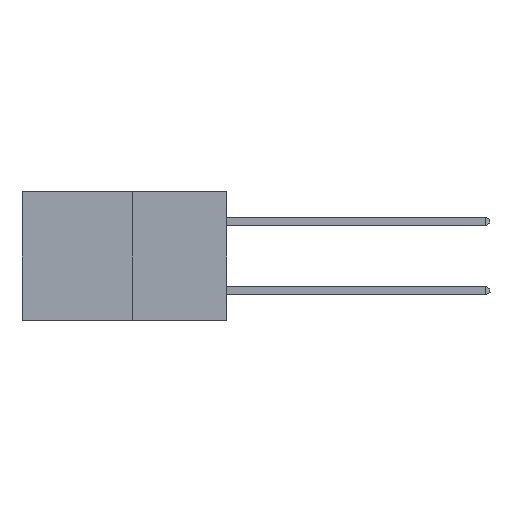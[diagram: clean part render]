
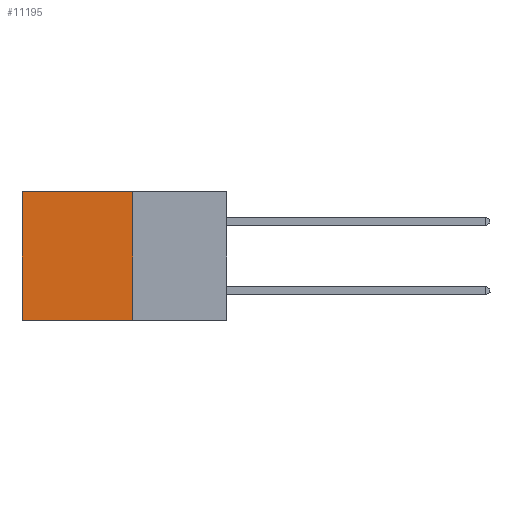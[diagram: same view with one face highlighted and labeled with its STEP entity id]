
A CAD part, left-side view. The second image highlights one B-rep face of the part: STEP entity #11195.
In plain terms, the highlighted planar face has unit normal (-1, 0, 0).
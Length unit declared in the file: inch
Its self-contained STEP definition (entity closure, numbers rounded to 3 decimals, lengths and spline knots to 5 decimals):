
#825 = ORIENTED_EDGE ( 'NONE', *, *, #18292, .T. ) ;
#1033 = LINE ( 'NONE', #4911, #9788 ) ;
#1078 = EDGE_CURVE ( 'NONE', #21351, #6214, #1033, .T. ) ;
#2439 = VERTEX_POINT ( 'NONE', #6594 ) ;
#2441 = LINE ( 'NONE', #10030, #19713 ) ;
#3381 = CARTESIAN_POINT ( 'NONE',  ( 0.277, 0.59, -0.37 ) ) ;
#4911 = CARTESIAN_POINT ( 'NONE',  ( 0.277, 0.27, -0.37 ) ) ;
#5107 = CARTESIAN_POINT ( 'NONE',  ( 0.277, 0.27, 0. ) ) ;
#5161 = DIRECTION ( 'NONE',  ( 0., 1., 0. ) ) ;
#5573 = EDGE_CURVE ( 'NONE', #21214, #2439, #19876, .T. ) ;
#6214 = VERTEX_POINT ( 'NONE', #7865 ) ;
#6594 = CARTESIAN_POINT ( 'NONE',  ( 0.277, 0.59, 0. ) ) ;
#7865 = CARTESIAN_POINT ( 'NONE',  ( 0.277, 0.59, -0.37 ) ) ;
#8168 = PLANE ( 'NONE',  #9071 ) ;
#9071 = AXIS2_PLACEMENT_3D ( 'NONE', #18413, #20121, #9875 ) ;
#9674 = ORIENTED_EDGE ( 'NONE', *, *, #5573, .T. ) ;
#9788 = VECTOR ( 'NONE', #16468, 39.37008 ) ;
#9875 = DIRECTION ( 'NONE',  ( 0., 0., -1. ) ) ;
#10030 = CARTESIAN_POINT ( 'NONE',  ( 0.277, 0.27, -0.37 ) ) ;
#10234 = VECTOR ( 'NONE', #5161, 39.37008 ) ;
#11195 = ADVANCED_FACE ( 'NONE', ( #18753 ), #8168, .F. ) ;
#12161 = DIRECTION ( 'NONE',  ( 0., 0., -1. ) ) ;
#12458 = CARTESIAN_POINT ( 'NONE',  ( 0.277, 0.27, 0. ) ) ;
#12824 = CARTESIAN_POINT ( 'NONE',  ( 0.277, 0.27, -0.37 ) ) ;
#13513 = ORIENTED_EDGE ( 'NONE', *, *, #1078, .F. ) ;
#16468 = DIRECTION ( 'NONE',  ( 0., 1., 0. ) ) ;
#18278 = EDGE_LOOP ( 'NONE', ( #825, #13513, #19864, #9674 ) ) ;
#18292 = EDGE_CURVE ( 'NONE', #2439, #6214, #18399, .T. ) ;
#18399 = LINE ( 'NONE', #3381, #21813 ) ;
#18413 = CARTESIAN_POINT ( 'NONE',  ( 0.277, 0.27, -0.37 ) ) ;
#18753 = FACE_OUTER_BOUND ( 'NONE', #18278, .T. ) ;
#18862 = EDGE_CURVE ( 'NONE', #21214, #21351, #2441, .T. ) ;
#19713 = VECTOR ( 'NONE', #20289, 39.37008 ) ;
#19864 = ORIENTED_EDGE ( 'NONE', *, *, #18862, .F. ) ;
#19876 = LINE ( 'NONE', #5107, #10234 ) ;
#20121 = DIRECTION ( 'NONE',  ( 1., 0., 0. ) ) ;
#20289 = DIRECTION ( 'NONE',  ( 0., 0., -1. ) ) ;
#21214 = VERTEX_POINT ( 'NONE', #12458 ) ;
#21351 = VERTEX_POINT ( 'NONE', #12824 ) ;
#21813 = VECTOR ( 'NONE', #12161, 39.37008 ) ;
